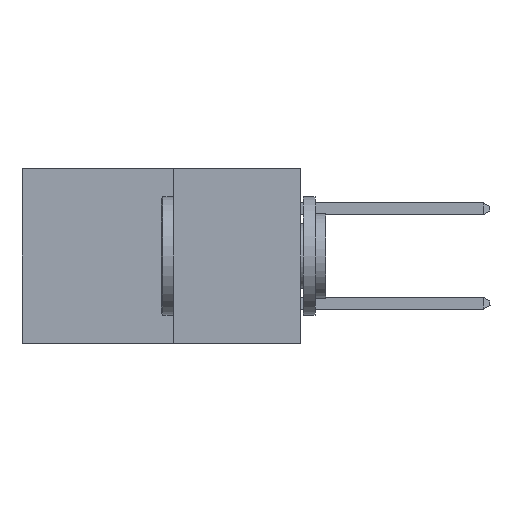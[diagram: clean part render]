
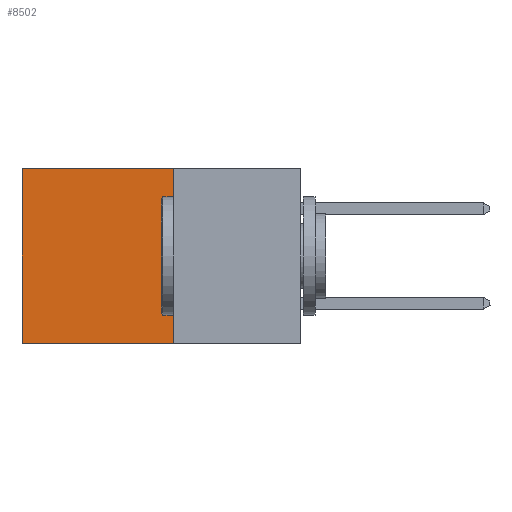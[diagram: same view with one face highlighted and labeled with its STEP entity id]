
A CAD part, left-side view. The second image highlights one B-rep face of the part: STEP entity #8502.
In plain terms, the highlighted planar face has unit normal (-1, 0, 0).
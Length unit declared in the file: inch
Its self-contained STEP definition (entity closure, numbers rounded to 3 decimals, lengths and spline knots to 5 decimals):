
#52 = VECTOR ( 'NONE', #14859, 39.37008 ) ;
#370 = EDGE_CURVE ( 'NONE', #13492, #5504, #14458, .T. ) ;
#3307 = DIRECTION ( 'NONE',  ( 1., 0., 0. ) ) ;
#3471 = CARTESIAN_POINT ( 'NONE',  ( 0.277, 0.27, 0. ) ) ;
#3939 = LINE ( 'NONE', #3471, #52 ) ;
#4622 = LINE ( 'NONE', #14400, #15878 ) ;
#4973 = VERTEX_POINT ( 'NONE', #10583 ) ;
#5002 = EDGE_CURVE ( 'NONE', #8086, #4973, #9893, .T. ) ;
#5504 = VERTEX_POINT ( 'NONE', #10388 ) ;
#6313 = ORIENTED_EDGE ( 'NONE', *, *, #9247, .T. ) ;
#6668 = CARTESIAN_POINT ( 'NONE',  ( 0.277, 0.59, 0. ) ) ;
#7715 = FACE_OUTER_BOUND ( 'NONE', #9624, .T. ) ;
#8086 = VERTEX_POINT ( 'NONE', #6668 ) ;
#8467 = ORIENTED_EDGE ( 'NONE', *, *, #370, .F. ) ;
#8502 = ADVANCED_FACE ( 'NONE', ( #7715 ), #11850, .F. ) ;
#8619 = ORIENTED_EDGE ( 'NONE', *, *, #5002, .T. ) ;
#8663 = DIRECTION ( 'NONE',  ( 0., 1., 0. ) ) ;
#8725 = DIRECTION ( 'NONE',  ( 0., 0., -1. ) ) ;
#8805 = CARTESIAN_POINT ( 'NONE',  ( 0.277, 0.27, -0.37 ) ) ;
#8963 = EDGE_CURVE ( 'NONE', #5504, #4973, #4622, .T. ) ;
#9247 = EDGE_CURVE ( 'NONE', #13492, #8086, #3939, .T. ) ;
#9624 = EDGE_LOOP ( 'NONE', ( #8619, #10922, #8467, #6313 ) ) ;
#9893 = LINE ( 'NONE', #13984, #13221 ) ;
#10388 = CARTESIAN_POINT ( 'NONE',  ( 0.277, 0.27, -0.37 ) ) ;
#10583 = CARTESIAN_POINT ( 'NONE',  ( 0.277, 0.59, -0.37 ) ) ;
#10922 = ORIENTED_EDGE ( 'NONE', *, *, #8963, .F. ) ;
#11064 = CARTESIAN_POINT ( 'NONE',  ( 0.277, 0.27, 0. ) ) ;
#11850 = PLANE ( 'NONE',  #17114 ) ;
#13221 = VECTOR ( 'NONE', #17251, 39.37008 ) ;
#13279 = DIRECTION ( 'NONE',  ( 0., 0., -1. ) ) ;
#13492 = VERTEX_POINT ( 'NONE', #11064 ) ;
#13984 = CARTESIAN_POINT ( 'NONE',  ( 0.277, 0.59, -0.37 ) ) ;
#14044 = VECTOR ( 'NONE', #8725, 39.37008 ) ;
#14400 = CARTESIAN_POINT ( 'NONE',  ( 0.277, 0.27, -0.37 ) ) ;
#14458 = LINE ( 'NONE', #8805, #14044 ) ;
#14859 = DIRECTION ( 'NONE',  ( 0., 1., 0. ) ) ;
#15878 = VECTOR ( 'NONE', #8663, 39.37008 ) ;
#17114 = AXIS2_PLACEMENT_3D ( 'NONE', #17366, #3307, #13279 ) ;
#17251 = DIRECTION ( 'NONE',  ( 0., 0., -1. ) ) ;
#17366 = CARTESIAN_POINT ( 'NONE',  ( 0.277, 0.27, -0.37 ) ) ;
